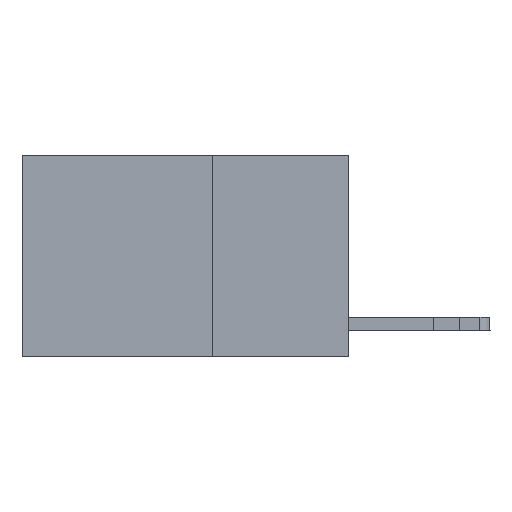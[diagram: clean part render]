
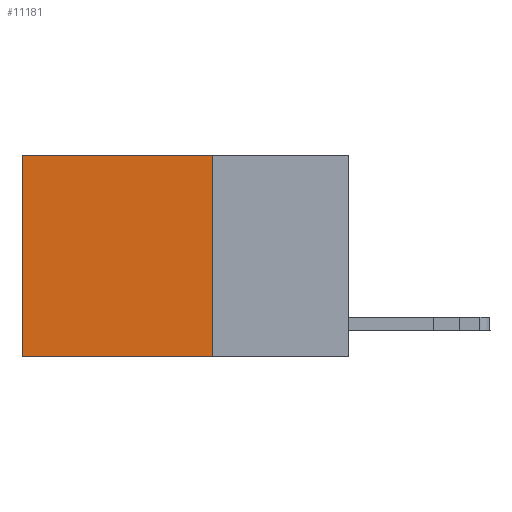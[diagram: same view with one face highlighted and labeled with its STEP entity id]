
A CAD part, left-side view. The second image highlights one B-rep face of the part: STEP entity #11181.
In plain terms, the highlighted planar face has unit normal (-1, 0, 0).
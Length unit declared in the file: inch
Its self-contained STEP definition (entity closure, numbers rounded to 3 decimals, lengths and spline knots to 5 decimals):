
#485 = CARTESIAN_POINT ( 'NONE',  ( 0.2625, 0.25, -0.37 ) ) ;
#792 = VERTEX_POINT ( 'NONE', #485 ) ;
#2785 = VECTOR ( 'NONE', #5642, 39.37008 ) ;
#3884 = EDGE_CURVE ( 'NONE', #7921, #4612, #6197, .T. ) ;
#4297 = CARTESIAN_POINT ( 'NONE',  ( 0.2625, 0.25, 0. ) ) ;
#4612 = VERTEX_POINT ( 'NONE', #10811 ) ;
#4907 = VECTOR ( 'NONE', #9760, 39.37008 ) ;
#5286 = VERTEX_POINT ( 'NONE', #14187 ) ;
#5311 = LINE ( 'NONE', #8533, #4907 ) ;
#5373 = EDGE_CURVE ( 'NONE', #792, #5286, #5570, .T. ) ;
#5427 = ORIENTED_EDGE ( 'NONE', *, *, #15593, .T. ) ;
#5570 = LINE ( 'NONE', #8069, #11940 ) ;
#5642 = DIRECTION ( 'NONE',  ( 0., 1., 0. ) ) ;
#6197 = LINE ( 'NONE', #15650, #2785 ) ;
#7453 = DIRECTION ( 'NONE',  ( 1., 0., 0. ) ) ;
#7475 = DIRECTION ( 'NONE',  ( 0., 0., -1. ) ) ;
#7921 = VERTEX_POINT ( 'NONE', #4297 ) ;
#8069 = CARTESIAN_POINT ( 'NONE',  ( 0.2625, 0.25, -0.37 ) ) ;
#8262 = FACE_OUTER_BOUND ( 'NONE', #14402, .T. ) ;
#8533 = CARTESIAN_POINT ( 'NONE',  ( 0.2625, 0.6, 0. ) ) ;
#9196 = ORIENTED_EDGE ( 'NONE', *, *, #3884, .T. ) ;
#9353 = DIRECTION ( 'NONE',  ( 0., 1., 0. ) ) ;
#9760 = DIRECTION ( 'NONE',  ( 0., 0., -1. ) ) ;
#9999 = CARTESIAN_POINT ( 'NONE',  ( 0.2625, 0.25, 0. ) ) ;
#10509 = VECTOR ( 'NONE', #7475, 39.37008 ) ;
#10768 = ORIENTED_EDGE ( 'NONE', *, *, #16381, .F. ) ;
#10811 = CARTESIAN_POINT ( 'NONE',  ( 0.2625, 0.6, 0. ) ) ;
#11181 = ADVANCED_FACE ( 'NONE', ( #8262 ), #12513, .F. ) ;
#11940 = VECTOR ( 'NONE', #9353, 39.37008 ) ;
#12513 = PLANE ( 'NONE',  #13143 ) ;
#13143 = AXIS2_PLACEMENT_3D ( 'NONE', #9999, #7453, #16217 ) ;
#13842 = LINE ( 'NONE', #16239, #10509 ) ;
#14187 = CARTESIAN_POINT ( 'NONE',  ( 0.2625, 0.6, -0.37 ) ) ;
#14402 = EDGE_LOOP ( 'NONE', ( #5427, #15848, #10768, #9196 ) ) ;
#15593 = EDGE_CURVE ( 'NONE', #4612, #5286, #5311, .T. ) ;
#15650 = CARTESIAN_POINT ( 'NONE',  ( 0.2625, 0.25, 0. ) ) ;
#15848 = ORIENTED_EDGE ( 'NONE', *, *, #5373, .F. ) ;
#16217 = DIRECTION ( 'NONE',  ( 0., 0., -1. ) ) ;
#16239 = CARTESIAN_POINT ( 'NONE',  ( 0.2625, 0.25, 0. ) ) ;
#16381 = EDGE_CURVE ( 'NONE', #7921, #792, #13842, .T. ) ;
